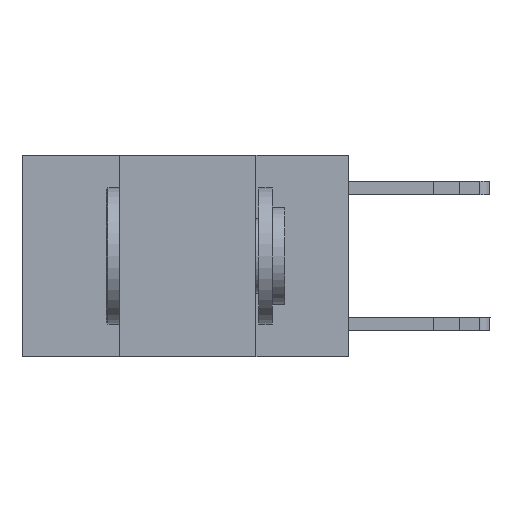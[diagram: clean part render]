
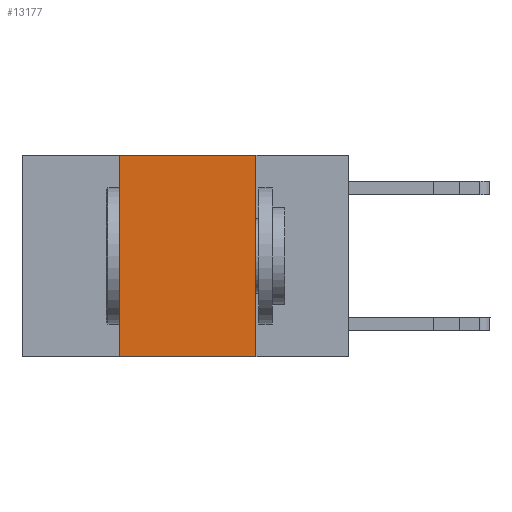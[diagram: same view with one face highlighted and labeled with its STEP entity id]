
A CAD part, left-side view. The second image highlights one B-rep face of the part: STEP entity #13177.
In plain terms, the highlighted planar face has unit normal (-1, 0, 0).
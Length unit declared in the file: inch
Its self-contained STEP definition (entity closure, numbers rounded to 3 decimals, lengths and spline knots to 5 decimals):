
#510 = CARTESIAN_POINT ( 'NONE',  ( 0., 0.42, 0. ) ) ;
#543 = VECTOR ( 'NONE', #1201, 39.37008 ) ;
#557 = LINE ( 'NONE', #610, #543 ) ;
#610 = CARTESIAN_POINT ( 'NONE',  ( 0., 0.17, 0. ) ) ;
#687 = CARTESIAN_POINT ( 'NONE',  ( 0., 0.17, -0.37 ) ) ;
#877 = EDGE_CURVE ( 'NONE', #7468, #2072, #20541, .T. ) ;
#1201 = DIRECTION ( 'NONE',  ( 0., 0., -1. ) ) ;
#2072 = VERTEX_POINT ( 'NONE', #510 ) ;
#2073 = EDGE_CURVE ( 'NONE', #8579, #15430, #557, .T. ) ;
#2313 = LINE ( 'NONE', #14722, #2462 ) ;
#2462 = VECTOR ( 'NONE', #9575, 39.37008 ) ;
#6546 = FACE_OUTER_BOUND ( 'NONE', #8051, .T. ) ;
#7468 = VERTEX_POINT ( 'NONE', #13162 ) ;
#8051 = EDGE_LOOP ( 'NONE', ( #11464, #12055, #12744, #13131 ) ) ;
#8579 = VERTEX_POINT ( 'NONE', #16730 ) ;
#9575 = DIRECTION ( 'NONE',  ( 0., -1., 0. ) ) ;
#10224 = CARTESIAN_POINT ( 'NONE',  ( 0., 0.6, 0. ) ) ;
#10227 = DIRECTION ( 'NONE',  ( 0., -1., 0. ) ) ;
#11464 = ORIENTED_EDGE ( 'NONE', *, *, #2073, .F. ) ;
#12055 = ORIENTED_EDGE ( 'NONE', *, *, #17883, .F. ) ;
#12636 = DIRECTION ( 'NONE',  ( 0., 0., -1. ) ) ;
#12642 = DIRECTION ( 'NONE',  ( 1., 0., 0. ) ) ;
#12665 = CARTESIAN_POINT ( 'NONE',  ( 0., 0.6, 0. ) ) ;
#12744 = ORIENTED_EDGE ( 'NONE', *, *, #877, .F. ) ;
#12803 = PLANE ( 'NONE',  #21672 ) ;
#13131 = ORIENTED_EDGE ( 'NONE', *, *, #21766, .T. ) ;
#13162 = CARTESIAN_POINT ( 'NONE',  ( 0., 0.42, -0.37 ) ) ;
#13177 = ADVANCED_FACE ( 'NONE', ( #6546 ), #12803, .F. ) ;
#14722 = CARTESIAN_POINT ( 'NONE',  ( 0., 0.6, -0.37 ) ) ;
#15430 = VERTEX_POINT ( 'NONE', #687 ) ;
#16730 = CARTESIAN_POINT ( 'NONE',  ( 0., 0.17, 0. ) ) ;
#17225 = DIRECTION ( 'NONE',  ( 0., 0., 1. ) ) ;
#17279 = CARTESIAN_POINT ( 'NONE',  ( 0., 0.42, 0. ) ) ;
#17883 = EDGE_CURVE ( 'NONE', #2072, #8579, #19901, .T. ) ;
#19865 = VECTOR ( 'NONE', #10227, 39.37008 ) ;
#19901 = LINE ( 'NONE', #10224, #19865 ) ;
#20326 = VECTOR ( 'NONE', #17225, 39.37008 ) ;
#20541 = LINE ( 'NONE', #17279, #20326 ) ;
#21672 = AXIS2_PLACEMENT_3D ( 'NONE', #12665, #12642, #12636 ) ;
#21766 = EDGE_CURVE ( 'NONE', #7468, #15430, #2313, .T. ) ;
